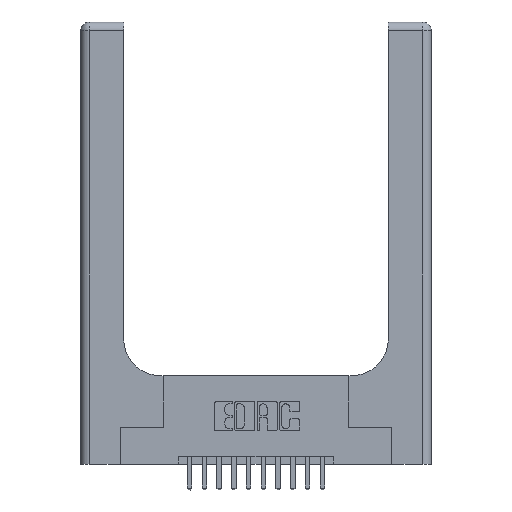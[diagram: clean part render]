
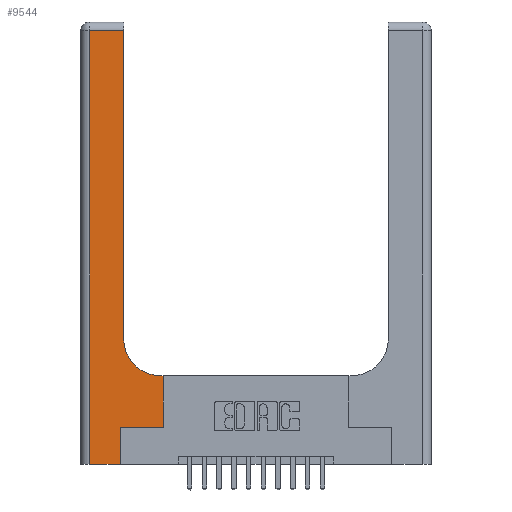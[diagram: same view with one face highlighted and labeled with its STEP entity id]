
A CAD part, top view. The second image highlights one B-rep face of the part: STEP entity #9544.
In plain terms, the highlighted planar face has unit normal (0, 0, 1).
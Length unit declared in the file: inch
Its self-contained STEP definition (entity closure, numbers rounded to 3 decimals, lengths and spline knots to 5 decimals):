
#234 = PLANE ( 'NONE',  #14501 ) ;
#351 = CARTESIAN_POINT ( 'NONE',  ( 0., 3., 0.37 ) ) ;
#513 = VECTOR ( 'NONE', #13308, 39.37008 ) ;
#647 = FACE_OUTER_BOUND ( 'NONE', #1909, .T. ) ;
#1066 = ORIENTED_EDGE ( 'NONE', *, *, #1411, .T. ) ;
#1340 = VECTOR ( 'NONE', #16081, 39.37008 ) ;
#1411 = EDGE_CURVE ( 'NONE', #1665, #15508, #14657, .T. ) ;
#1608 = ORIENTED_EDGE ( 'NONE', *, *, #7487, .T. ) ;
#1618 = VERTEX_POINT ( 'NONE', #12907 ) ;
#1638 = DIRECTION ( 'NONE',  ( -1., 0., 0. ) ) ;
#1665 = VERTEX_POINT ( 'NONE', #2262 ) ;
#1901 = CARTESIAN_POINT ( 'NONE',  ( 0.5415, 0.85, 0.37 ) ) ;
#1909 = EDGE_LOOP ( 'NONE', ( #13488, #8814, #16669, #1066, #9455, #6943, #14080, #1608, #12686 ) ) ;
#1982 = VERTEX_POINT ( 'NONE', #14258 ) ;
#2262 = CARTESIAN_POINT ( 'NONE',  ( 0.06, 0., 0.37 ) ) ;
#2512 = CARTESIAN_POINT ( 'NONE',  ( 0.5585, 0.25, 0.37 ) ) ;
#3258 = DIRECTION ( 'NONE',  ( 1., 0., 0. ) ) ;
#3329 = VECTOR ( 'NONE', #7309, 39.37008 ) ;
#3885 = DIRECTION ( 'NONE',  ( 0., 1., 0. ) ) ;
#4628 = AXIS2_PLACEMENT_3D ( 'NONE', #1901, #7305, #3258 ) ;
#4831 = EDGE_CURVE ( 'NONE', #16131, #15432, #5048, .T. ) ;
#4954 = VECTOR ( 'NONE', #7188, 39.37008 ) ;
#5034 = EDGE_CURVE ( 'NONE', #15508, #11145, #8432, .T. ) ;
#5048 = LINE ( 'NONE', #2512, #14922 ) ;
#5377 = CARTESIAN_POINT ( 'NONE',  ( 0.06, 3., 0.37 ) ) ;
#5540 = EDGE_CURVE ( 'NONE', #11145, #16131, #8203, .T. ) ;
#5816 = CARTESIAN_POINT ( 'NONE',  ( 0., 0., 0.37 ) ) ;
#5835 = LINE ( 'NONE', #7709, #6047 ) ;
#5950 = DIRECTION ( 'NONE',  ( 0., 1., 0. ) ) ;
#6020 = LINE ( 'NONE', #8143, #513 ) ;
#6047 = VECTOR ( 'NONE', #15701, 39.37008 ) ;
#6943 = ORIENTED_EDGE ( 'NONE', *, *, #5540, .T. ) ;
#7188 = DIRECTION ( 'NONE',  ( 1., 0., 0. ) ) ;
#7305 = DIRECTION ( 'NONE',  ( 0., 0., -1. ) ) ;
#7309 = DIRECTION ( 'NONE',  ( 1., 0., 0. ) ) ;
#7412 = EDGE_CURVE ( 'NONE', #1618, #1982, #8989, .T. ) ;
#7487 = EDGE_CURVE ( 'NONE', #15432, #16139, #6020, .T. ) ;
#7709 = CARTESIAN_POINT ( 'NONE',  ( 0., 2.94, 0.37 ) ) ;
#8143 = CARTESIAN_POINT ( 'NONE',  ( 0.2915, 0.6, 0.37 ) ) ;
#8203 = LINE ( 'NONE', #11240, #3329 ) ;
#8345 = DIRECTION ( 'NONE',  ( 0., 0., -1. ) ) ;
#8432 = LINE ( 'NONE', #9891, #14520 ) ;
#8435 = VERTEX_POINT ( 'NONE', #12911 ) ;
#8814 = ORIENTED_EDGE ( 'NONE', *, *, #11534, .T. ) ;
#8989 = LINE ( 'NONE', #14841, #1340 ) ;
#9455 = ORIENTED_EDGE ( 'NONE', *, *, #5034, .T. ) ;
#9544 = ADVANCED_FACE ( 'NONE', ( #647 ), #234, .F. ) ;
#9589 = CARTESIAN_POINT ( 'NONE',  ( 0.5415, 0.6, 0.37 ) ) ;
#9891 = CARTESIAN_POINT ( 'NONE',  ( 0.269, 0., 0.37 ) ) ;
#10764 = CARTESIAN_POINT ( 'NONE',  ( 0.5585, 0.25, 0.37 ) ) ;
#10879 = LINE ( 'NONE', #5377, #12287 ) ;
#11145 = VERTEX_POINT ( 'NONE', #15011 ) ;
#11240 = CARTESIAN_POINT ( 'NONE',  ( 0.269, 0.25, 0.37 ) ) ;
#11534 = EDGE_CURVE ( 'NONE', #1982, #8435, #5835, .T. ) ;
#12287 = VECTOR ( 'NONE', #16144, 39.37008 ) ;
#12686 = ORIENTED_EDGE ( 'NONE', *, *, #15782, .T. ) ;
#12907 = CARTESIAN_POINT ( 'NONE',  ( 0.2915, 0.85, 0.37 ) ) ;
#12911 = CARTESIAN_POINT ( 'NONE',  ( 0.06, 2.94, 0.37 ) ) ;
#13308 = DIRECTION ( 'NONE',  ( -1., 0., 0. ) ) ;
#13488 = ORIENTED_EDGE ( 'NONE', *, *, #7412, .T. ) ;
#14080 = ORIENTED_EDGE ( 'NONE', *, *, #4831, .T. ) ;
#14258 = CARTESIAN_POINT ( 'NONE',  ( 0.2915, 2.94, 0.37 ) ) ;
#14501 = AXIS2_PLACEMENT_3D ( 'NONE', #351, #8345, #1638 ) ;
#14520 = VECTOR ( 'NONE', #5950, 39.37008 ) ;
#14657 = LINE ( 'NONE', #5816, #4954 ) ;
#14768 = CIRCLE ( 'NONE', #4628, 0.25 ) ;
#14841 = CARTESIAN_POINT ( 'NONE',  ( 0.2915, 3., 0.37 ) ) ;
#14922 = VECTOR ( 'NONE', #3885, 39.37008 ) ;
#15011 = CARTESIAN_POINT ( 'NONE',  ( 0.269, 0.25, 0.37 ) ) ;
#15432 = VERTEX_POINT ( 'NONE', #17049 ) ;
#15508 = VERTEX_POINT ( 'NONE', #17420 ) ;
#15701 = DIRECTION ( 'NONE',  ( -1., 0., 0. ) ) ;
#15782 = EDGE_CURVE ( 'NONE', #16139, #1618, #14768, .T. ) ;
#16081 = DIRECTION ( 'NONE',  ( 0., 1., 0. ) ) ;
#16131 = VERTEX_POINT ( 'NONE', #10764 ) ;
#16139 = VERTEX_POINT ( 'NONE', #9589 ) ;
#16144 = DIRECTION ( 'NONE',  ( 0., -1., 0. ) ) ;
#16669 = ORIENTED_EDGE ( 'NONE', *, *, #17091, .T. ) ;
#17049 = CARTESIAN_POINT ( 'NONE',  ( 0.5585, 0.6, 0.37 ) ) ;
#17091 = EDGE_CURVE ( 'NONE', #8435, #1665, #10879, .T. ) ;
#17420 = CARTESIAN_POINT ( 'NONE',  ( 0.269, 0., 0.37 ) ) ;
